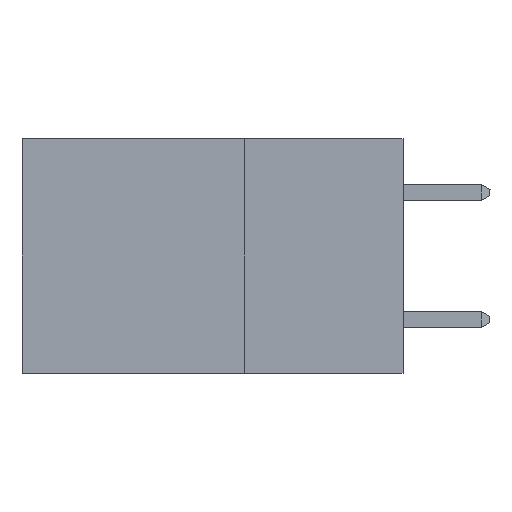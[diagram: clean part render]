
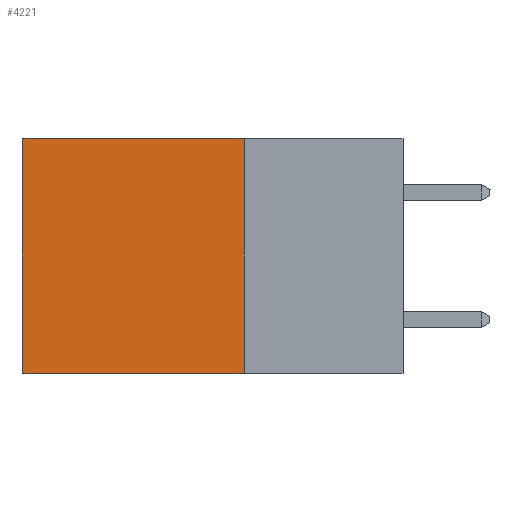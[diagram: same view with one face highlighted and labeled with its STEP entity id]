
A CAD part, left-side view. The second image highlights one B-rep face of the part: STEP entity #4221.
In plain terms, the highlighted planar face has unit normal (-1, 0, 0).
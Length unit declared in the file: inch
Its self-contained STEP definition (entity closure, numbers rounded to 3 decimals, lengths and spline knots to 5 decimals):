
#1617 = ORIENTED_EDGE ( 'NONE', *, *, #3732, .T. ) ;
#2022 = LINE ( 'NONE', #3993, #20043 ) ;
#2640 = EDGE_LOOP ( 'NONE', ( #9445, #19336, #10486, #1617 ) ) ;
#2889 = AXIS2_PLACEMENT_3D ( 'NONE', #6090, #4395, #7740 ) ;
#3429 = CARTESIAN_POINT ( 'NONE',  ( 0.2875, 0.25, 0. ) ) ;
#3732 = EDGE_CURVE ( 'NONE', #17410, #6786, #18063, .T. ) ;
#3993 = CARTESIAN_POINT ( 'NONE',  ( 0.2875, 0.25, -0.37 ) ) ;
#4221 = ADVANCED_FACE ( 'NONE', ( #13349 ), #13314, .F. ) ;
#4378 = EDGE_CURVE ( 'NONE', #5161, #18779, #2022, .T. ) ;
#4395 = DIRECTION ( 'NONE',  ( 1., 0., 0. ) ) ;
#4870 = CARTESIAN_POINT ( 'NONE',  ( 0.2875, 0.6, -0.37 ) ) ;
#5161 = VERTEX_POINT ( 'NONE', #20472 ) ;
#5188 = EDGE_CURVE ( 'NONE', #6786, #18779, #9231, .T. ) ;
#6090 = CARTESIAN_POINT ( 'NONE',  ( 0.2875, 0.25, 0. ) ) ;
#6633 = VECTOR ( 'NONE', #18918, 39.37008 ) ;
#6786 = VERTEX_POINT ( 'NONE', #9702 ) ;
#7740 = DIRECTION ( 'NONE',  ( 0., 0., -1. ) ) ;
#9231 = LINE ( 'NONE', #12303, #6633 ) ;
#9391 = EDGE_CURVE ( 'NONE', #17410, #5161, #11597, .T. ) ;
#9445 = ORIENTED_EDGE ( 'NONE', *, *, #5188, .T. ) ;
#9702 = CARTESIAN_POINT ( 'NONE',  ( 0.2875, 0.6, 0. ) ) ;
#10486 = ORIENTED_EDGE ( 'NONE', *, *, #9391, .F. ) ;
#11597 = LINE ( 'NONE', #15827, #15464 ) ;
#12029 = CARTESIAN_POINT ( 'NONE',  ( 0.2875, 0.25, 0. ) ) ;
#12131 = VECTOR ( 'NONE', #13267, 39.37008 ) ;
#12303 = CARTESIAN_POINT ( 'NONE',  ( 0.2875, 0.6, 0. ) ) ;
#13267 = DIRECTION ( 'NONE',  ( 0., 1., 0. ) ) ;
#13314 = PLANE ( 'NONE',  #2889 ) ;
#13349 = FACE_OUTER_BOUND ( 'NONE', #2640, .T. ) ;
#15464 = VECTOR ( 'NONE', #19148, 39.37008 ) ;
#15492 = DIRECTION ( 'NONE',  ( 0., 1., 0. ) ) ;
#15827 = CARTESIAN_POINT ( 'NONE',  ( 0.2875, 0.25, 0. ) ) ;
#17410 = VERTEX_POINT ( 'NONE', #3429 ) ;
#18063 = LINE ( 'NONE', #12029, #12131 ) ;
#18779 = VERTEX_POINT ( 'NONE', #4870 ) ;
#18918 = DIRECTION ( 'NONE',  ( 0., 0., -1. ) ) ;
#19148 = DIRECTION ( 'NONE',  ( 0., 0., -1. ) ) ;
#19336 = ORIENTED_EDGE ( 'NONE', *, *, #4378, .F. ) ;
#20043 = VECTOR ( 'NONE', #15492, 39.37008 ) ;
#20472 = CARTESIAN_POINT ( 'NONE',  ( 0.2875, 0.25, -0.37 ) ) ;
